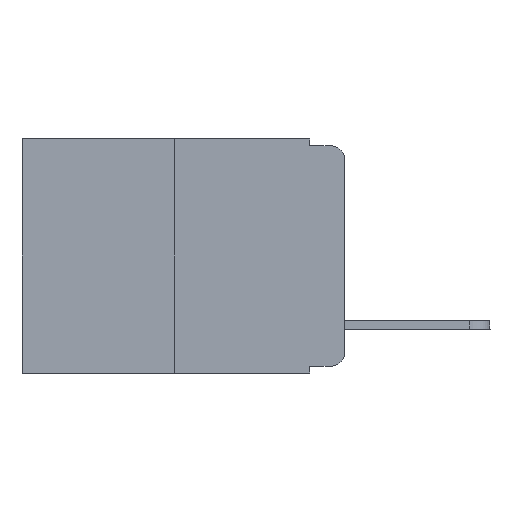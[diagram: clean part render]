
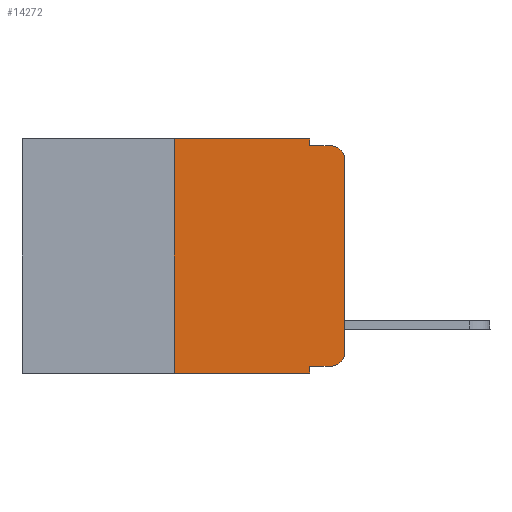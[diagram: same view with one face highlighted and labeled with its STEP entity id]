
A CAD part, left-side view. The second image highlights one B-rep face of the part: STEP entity #14272.
In plain terms, the highlighted planar face has unit normal (-1, 0, 0).
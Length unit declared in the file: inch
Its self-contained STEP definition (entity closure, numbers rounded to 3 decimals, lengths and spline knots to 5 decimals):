
#194 = CARTESIAN_POINT ( 'NONE',  ( 0., 0., -0.313 ) ) ;
#200 = DIRECTION ( 'NONE',  ( 0., 0., -1. ) ) ;
#373 = EDGE_CURVE ( 'NONE', #12370, #10897, #3979, .T. ) ;
#590 = CARTESIAN_POINT ( 'NONE',  ( 0., 0.473, -0.343 ) ) ;
#684 = CARTESIAN_POINT ( 'NONE',  ( 0., 0.473, 0. ) ) ;
#836 = VECTOR ( 'NONE', #10116, 39.37008 ) ;
#1089 = EDGE_CURVE ( 'NONE', #10897, #11990, #2329, .T. ) ;
#1158 = ORIENTED_EDGE ( 'NONE', *, *, #5762, .T. ) ;
#1521 = DIRECTION ( 'NONE',  ( 0., -1., 0. ) ) ;
#1639 = DIRECTION ( 'NONE',  ( 0., 0., 1. ) ) ;
#1734 = PLANE ( 'NONE',  #15386 ) ;
#1978 = DIRECTION ( 'NONE',  ( 0., 0., -1. ) ) ;
#2081 = DIRECTION ( 'NONE',  ( 0., -1., 0. ) ) ;
#2240 = ORIENTED_EDGE ( 'NONE', *, *, #15862, .F. ) ;
#2329 = LINE ( 'NONE', #13349, #5705 ) ;
#2392 = EDGE_CURVE ( 'NONE', #2832, #12711, #7649, .T. ) ;
#2770 = AXIS2_PLACEMENT_3D ( 'NONE', #12435, #2871, #200 ) ;
#2832 = VERTEX_POINT ( 'NONE', #194 ) ;
#2871 = DIRECTION ( 'NONE',  ( -1., 0., 0. ) ) ;
#3001 = LINE ( 'NONE', #15423, #11799 ) ;
#3044 = ORIENTED_EDGE ( 'NONE', *, *, #14061, .F. ) ;
#3335 = VERTEX_POINT ( 'NONE', #9123 ) ;
#3462 = ORIENTED_EDGE ( 'NONE', *, *, #14181, .T. ) ;
#3611 = CARTESIAN_POINT ( 'NONE',  ( 0., 0.051, 0. ) ) ;
#3785 = VERTEX_POINT ( 'NONE', #9638 ) ;
#3979 = LINE ( 'NONE', #9051, #10029 ) ;
#4151 = VECTOR ( 'NONE', #2081, 39.37008 ) ;
#4474 = CARTESIAN_POINT ( 'NONE',  ( 0., 0.25, 0. ) ) ;
#4576 = CARTESIAN_POINT ( 'NONE',  ( 0., 0.051, -0.333 ) ) ;
#4905 = CARTESIAN_POINT ( 'NONE',  ( 0., 0., -0.03 ) ) ;
#4980 = ORIENTED_EDGE ( 'NONE', *, *, #373, .F. ) ;
#5225 = ORIENTED_EDGE ( 'NONE', *, *, #2392, .T. ) ;
#5563 = ORIENTED_EDGE ( 'NONE', *, *, #13421, .T. ) ;
#5705 = VECTOR ( 'NONE', #9572, 39.37008 ) ;
#5762 = EDGE_CURVE ( 'NONE', #12711, #10088, #10460, .T. ) ;
#6132 = CIRCLE ( 'NONE', #2770, 0.02 ) ;
#6184 = VERTEX_POINT ( 'NONE', #9274 ) ;
#6538 = CARTESIAN_POINT ( 'NONE',  ( 0., 0., 0. ) ) ;
#6551 = LINE ( 'NONE', #14817, #11454 ) ;
#6610 = CARTESIAN_POINT ( 'NONE',  ( 0., 0.02, -0.333 ) ) ;
#7169 = LINE ( 'NONE', #3611, #15922 ) ;
#7649 = LINE ( 'NONE', #6538, #836 ) ;
#7938 = EDGE_CURVE ( 'NONE', #6184, #10088, #6551, .T. ) ;
#7963 = DIRECTION ( 'NONE',  ( 1., 0., 0. ) ) ;
#8520 = ORIENTED_EDGE ( 'NONE', *, *, #1089, .F. ) ;
#9051 = CARTESIAN_POINT ( 'NONE',  ( 0., 0.25, 0. ) ) ;
#9123 = CARTESIAN_POINT ( 'NONE',  ( 0., 0.051, -0.333 ) ) ;
#9133 = CARTESIAN_POINT ( 'NONE',  ( 0., 0.051, 0. ) ) ;
#9274 = CARTESIAN_POINT ( 'NONE',  ( 0., 0.051, -0.01 ) ) ;
#9572 = DIRECTION ( 'NONE',  ( 0., -1., 0. ) ) ;
#9638 = CARTESIAN_POINT ( 'NONE',  ( 0., 0.051, -0.343 ) ) ;
#10029 = VECTOR ( 'NONE', #1639, 39.37008 ) ;
#10088 = VERTEX_POINT ( 'NONE', #13182 ) ;
#10116 = DIRECTION ( 'NONE',  ( 0., 0., 1. ) ) ;
#10404 = CARTESIAN_POINT ( 'NONE',  ( 0., 0.02, -0.03 ) ) ;
#10460 = CIRCLE ( 'NONE', #14601, 0.02 ) ;
#10568 = LINE ( 'NONE', #590, #11776 ) ;
#10897 = VERTEX_POINT ( 'NONE', #4474 ) ;
#11454 = VECTOR ( 'NONE', #1521, 39.37008 ) ;
#11650 = VERTEX_POINT ( 'NONE', #6610 ) ;
#11713 = FACE_OUTER_BOUND ( 'NONE', #14273, .T. ) ;
#11729 = EDGE_CURVE ( 'NONE', #3335, #11650, #14243, .T. ) ;
#11758 = ORIENTED_EDGE ( 'NONE', *, *, #11729, .T. ) ;
#11776 = VECTOR ( 'NONE', #15181, 39.37008 ) ;
#11799 = VECTOR ( 'NONE', #14039, 39.37008 ) ;
#11990 = VERTEX_POINT ( 'NONE', #9133 ) ;
#12006 = DIRECTION ( 'NONE',  ( 0., 0., -1. ) ) ;
#12370 = VERTEX_POINT ( 'NONE', #15133 ) ;
#12435 = CARTESIAN_POINT ( 'NONE',  ( 0., 0.02, -0.313 ) ) ;
#12711 = VERTEX_POINT ( 'NONE', #4905 ) ;
#13182 = CARTESIAN_POINT ( 'NONE',  ( 0., 0.02, -0.01 ) ) ;
#13349 = CARTESIAN_POINT ( 'NONE',  ( 0., 0.473, 0. ) ) ;
#13421 = EDGE_CURVE ( 'NONE', #12370, #3785, #10568, .T. ) ;
#14039 = DIRECTION ( 'NONE',  ( 0., 0., -1. ) ) ;
#14061 = EDGE_CURVE ( 'NONE', #11990, #6184, #7169, .T. ) ;
#14101 = ORIENTED_EDGE ( 'NONE', *, *, #7938, .F. ) ;
#14181 = EDGE_CURVE ( 'NONE', #11650, #2832, #6132, .T. ) ;
#14243 = LINE ( 'NONE', #4576, #4151 ) ;
#14272 = ADVANCED_FACE ( 'NONE', ( #11713 ), #1734, .F. ) ;
#14273 = EDGE_LOOP ( 'NONE', ( #5225, #1158, #14101, #3044, #8520, #4980, #5563, #2240, #11758, #3462 ) ) ;
#14601 = AXIS2_PLACEMENT_3D ( 'NONE', #10404, #15333, #12006 ) ;
#14817 = CARTESIAN_POINT ( 'NONE',  ( 0., 0.051, -0.01 ) ) ;
#15133 = CARTESIAN_POINT ( 'NONE',  ( 0., 0.25, -0.343 ) ) ;
#15181 = DIRECTION ( 'NONE',  ( 0., -1., 0. ) ) ;
#15333 = DIRECTION ( 'NONE',  ( -1., 0., 0. ) ) ;
#15386 = AXIS2_PLACEMENT_3D ( 'NONE', #684, #7963, #1978 ) ;
#15423 = CARTESIAN_POINT ( 'NONE',  ( 0., 0.051, 0. ) ) ;
#15862 = EDGE_CURVE ( 'NONE', #3335, #3785, #3001, .T. ) ;
#15922 = VECTOR ( 'NONE', #15927, 39.37008 ) ;
#15927 = DIRECTION ( 'NONE',  ( 0., 0., -1. ) ) ;
